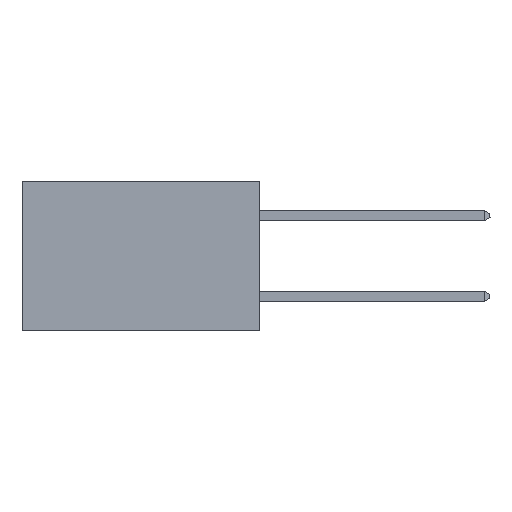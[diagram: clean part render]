
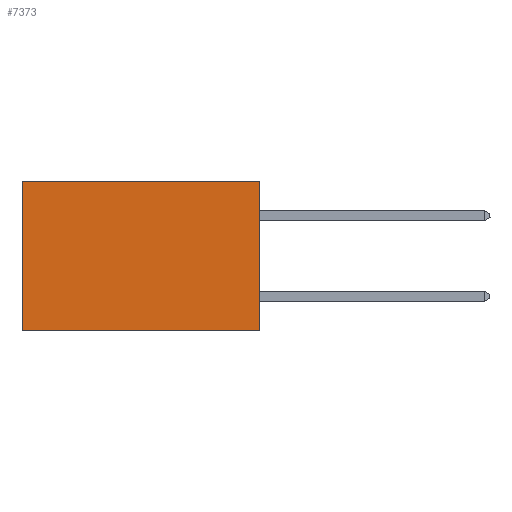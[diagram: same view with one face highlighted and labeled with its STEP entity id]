
A CAD part, left-side view. The second image highlights one B-rep face of the part: STEP entity #7373.
In plain terms, the highlighted planar face has unit normal (-1, 0, 0).
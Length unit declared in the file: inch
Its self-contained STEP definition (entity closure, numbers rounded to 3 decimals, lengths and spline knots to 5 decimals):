
#33 = DIRECTION ( 'NONE',  ( 0., 0., -1. ) ) ;
#78 = CARTESIAN_POINT ( 'NONE',  ( 0.277, 0., -0.37 ) ) ;
#107 = CARTESIAN_POINT ( 'NONE',  ( 0.277, 0., 0. ) ) ;
#143 = VERTEX_POINT ( 'NONE', #9871 ) ;
#1348 = VECTOR ( 'NONE', #12851, 39.37008 ) ;
#1424 = DIRECTION ( 'NONE',  ( 0., 1., 0. ) ) ;
#1824 = LINE ( 'NONE', #78, #14726 ) ;
#2478 = CARTESIAN_POINT ( 'NONE',  ( 0.277, 0.59, 0. ) ) ;
#4240 = VECTOR ( 'NONE', #19527, 39.37008 ) ;
#4312 = ORIENTED_EDGE ( 'NONE', *, *, #6011, .F. ) ;
#4586 = VECTOR ( 'NONE', #1424, 39.37008 ) ;
#4698 = VERTEX_POINT ( 'NONE', #107 ) ;
#6011 = EDGE_CURVE ( 'NONE', #4698, #143, #1824, .T. ) ;
#7373 = ADVANCED_FACE ( 'NONE', ( #8379 ), #13858, .F. ) ;
#8379 = FACE_OUTER_BOUND ( 'NONE', #13918, .T. ) ;
#8876 = CARTESIAN_POINT ( 'NONE',  ( 0.277, 0.59, -0.37 ) ) ;
#9871 = CARTESIAN_POINT ( 'NONE',  ( 0.277, 0., -0.37 ) ) ;
#10066 = AXIS2_PLACEMENT_3D ( 'NONE', #13856, #13834, #13832 ) ;
#10771 = CARTESIAN_POINT ( 'NONE',  ( 0.277, 0., -0.37 ) ) ;
#12851 = DIRECTION ( 'NONE',  ( 0., 1., 0. ) ) ;
#13832 = DIRECTION ( 'NONE',  ( 0., 0., -1. ) ) ;
#13834 = DIRECTION ( 'NONE',  ( 1., 0., 0. ) ) ;
#13856 = CARTESIAN_POINT ( 'NONE',  ( 0.277, 0., -0.37 ) ) ;
#13858 = PLANE ( 'NONE',  #10066 ) ;
#13918 = EDGE_LOOP ( 'NONE', ( #17808, #19229, #4312, #14541 ) ) ;
#14063 = EDGE_CURVE ( 'NONE', #4698, #16354, #16840, .T. ) ;
#14225 = VERTEX_POINT ( 'NONE', #14877 ) ;
#14293 = EDGE_CURVE ( 'NONE', #16354, #14225, #16114, .T. ) ;
#14485 = CARTESIAN_POINT ( 'NONE',  ( 0.277, 0., 0. ) ) ;
#14541 = ORIENTED_EDGE ( 'NONE', *, *, #14063, .T. ) ;
#14726 = VECTOR ( 'NONE', #33, 39.37008 ) ;
#14877 = CARTESIAN_POINT ( 'NONE',  ( 0.277, 0.59, -0.37 ) ) ;
#16114 = LINE ( 'NONE', #8876, #4240 ) ;
#16354 = VERTEX_POINT ( 'NONE', #2478 ) ;
#16840 = LINE ( 'NONE', #14485, #1348 ) ;
#17808 = ORIENTED_EDGE ( 'NONE', *, *, #14293, .T. ) ;
#18529 = EDGE_CURVE ( 'NONE', #143, #14225, #19938, .T. ) ;
#19229 = ORIENTED_EDGE ( 'NONE', *, *, #18529, .F. ) ;
#19527 = DIRECTION ( 'NONE',  ( 0., 0., -1. ) ) ;
#19938 = LINE ( 'NONE', #10771, #4586 ) ;
